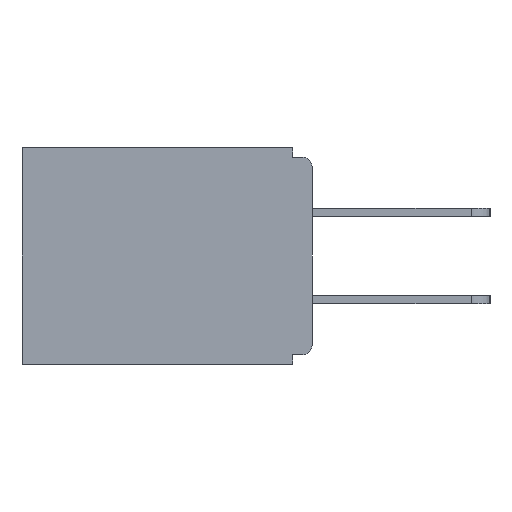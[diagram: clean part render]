
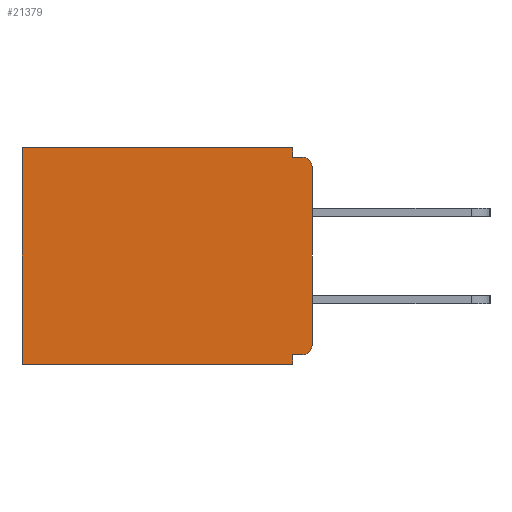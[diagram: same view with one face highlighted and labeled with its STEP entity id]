
A CAD part, left-side view. The second image highlights one B-rep face of the part: STEP entity #21379.
In plain terms, the highlighted planar face has unit normal (-1, 0, 0).
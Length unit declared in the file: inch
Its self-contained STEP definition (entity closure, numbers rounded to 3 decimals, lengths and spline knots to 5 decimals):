
#298 = VERTEX_POINT ( 'NONE', #12669 ) ;
#305 = DIRECTION ( 'NONE',  ( 0., 1., 0. ) ) ;
#724 = EDGE_CURVE ( 'NONE', #17799, #19816, #5233, .T. ) ;
#803 = AXIS2_PLACEMENT_3D ( 'NONE', #21367, #6289, #8257 ) ;
#1035 = DIRECTION ( 'NONE',  ( 0., 0., -1. ) ) ;
#2057 = CARTESIAN_POINT ( 'NONE',  ( 0.298, 0.031, -0.343 ) ) ;
#2880 = VECTOR ( 'NONE', #20160, 39.37008 ) ;
#3311 = DIRECTION ( 'NONE',  ( 0., 0., -1. ) ) ;
#3341 = DIRECTION ( 'NONE',  ( 0., 0., -1. ) ) ;
#4679 = VECTOR ( 'NONE', #11128, 39.37008 ) ;
#5233 = LINE ( 'NONE', #23841, #2880 ) ;
#5255 = CARTESIAN_POINT ( 'NONE',  ( 0.298, 0., 0. ) ) ;
#5290 = DIRECTION ( 'NONE',  ( 0., 0., -1. ) ) ;
#5450 = VECTOR ( 'NONE', #22810, 39.37008 ) ;
#5525 = EDGE_CURVE ( 'NONE', #14277, #6176, #12994, .T. ) ;
#5656 = VECTOR ( 'NONE', #10383, 39.37008 ) ;
#6069 = CARTESIAN_POINT ( 'NONE',  ( 0.298, 0.031, -0.015 ) ) ;
#6142 = LINE ( 'NONE', #14630, #7936 ) ;
#6176 = VERTEX_POINT ( 'NONE', #13397 ) ;
#6250 = EDGE_CURVE ( 'NONE', #19816, #13622, #6320, .T. ) ;
#6289 = DIRECTION ( 'NONE',  ( -1., 0., 0. ) ) ;
#6320 = LINE ( 'NONE', #11673, #5450 ) ;
#6567 = CARTESIAN_POINT ( 'NONE',  ( 0.298, 0.015, -0.328 ) ) ;
#6892 = ORIENTED_EDGE ( 'NONE', *, *, #5525, .T. ) ;
#7248 = CIRCLE ( 'NONE', #803, 0.015 ) ;
#7365 = DIRECTION ( 'NONE',  ( 0., 0., -1. ) ) ;
#7936 = VECTOR ( 'NONE', #5290, 39.37008 ) ;
#8257 = DIRECTION ( 'NONE',  ( 0., 0., -1. ) ) ;
#8286 = AXIS2_PLACEMENT_3D ( 'NONE', #5255, #8669, #3311 ) ;
#8337 = ORIENTED_EDGE ( 'NONE', *, *, #14405, .T. ) ;
#8435 = EDGE_CURVE ( 'NONE', #10183, #6176, #18971, .T. ) ;
#8669 = DIRECTION ( 'NONE',  ( 1., 0., 0. ) ) ;
#9319 = VERTEX_POINT ( 'NONE', #6567 ) ;
#9611 = ORIENTED_EDGE ( 'NONE', *, *, #6250, .F. ) ;
#9703 = CARTESIAN_POINT ( 'NONE',  ( 0.298, 0.46, 0. ) ) ;
#9891 = CARTESIAN_POINT ( 'NONE',  ( 0.298, 0.031, 0. ) ) ;
#10083 = VERTEX_POINT ( 'NONE', #23660 ) ;
#10183 = VERTEX_POINT ( 'NONE', #2057 ) ;
#10383 = DIRECTION ( 'NONE',  ( 0., 1., 0. ) ) ;
#10461 = DIRECTION ( 'NONE',  ( -1., 0., 0. ) ) ;
#11120 = LINE ( 'NONE', #22189, #21811 ) ;
#11128 = DIRECTION ( 'NONE',  ( 0., 1., 0. ) ) ;
#11460 = ORIENTED_EDGE ( 'NONE', *, *, #12858, .T. ) ;
#11673 = CARTESIAN_POINT ( 'NONE',  ( 0.298, 0., -0.015 ) ) ;
#11768 = EDGE_LOOP ( 'NONE', ( #15242, #9611, #22030, #11460, #6892, #17866, #12797, #11913, #8337, #17191 ) ) ;
#11913 = ORIENTED_EDGE ( 'NONE', *, *, #21423, .F. ) ;
#12168 = CARTESIAN_POINT ( 'NONE',  ( 0.298, 0.015, -0.03 ) ) ;
#12349 = CIRCLE ( 'NONE', #21362, 0.015 ) ;
#12669 = CARTESIAN_POINT ( 'NONE',  ( 0.298, 0., -0.03 ) ) ;
#12797 = ORIENTED_EDGE ( 'NONE', *, *, #12963, .F. ) ;
#12858 = EDGE_CURVE ( 'NONE', #17799, #14277, #20676, .T. ) ;
#12963 = EDGE_CURVE ( 'NONE', #14207, #10183, #11120, .T. ) ;
#12994 = LINE ( 'NONE', #18427, #23477 ) ;
#13124 = CARTESIAN_POINT ( 'NONE',  ( 0.298, 0.031, -0.328 ) ) ;
#13397 = CARTESIAN_POINT ( 'NONE',  ( 0.298, 0.46, -0.343 ) ) ;
#13405 = FACE_OUTER_BOUND ( 'NONE', #11768, .T. ) ;
#13622 = VERTEX_POINT ( 'NONE', #22935 ) ;
#14207 = VERTEX_POINT ( 'NONE', #13124 ) ;
#14277 = VERTEX_POINT ( 'NONE', #9703 ) ;
#14405 = EDGE_CURVE ( 'NONE', #9319, #10083, #7248, .T. ) ;
#14630 = CARTESIAN_POINT ( 'NONE',  ( 0.298, 0., 0. ) ) ;
#15242 = ORIENTED_EDGE ( 'NONE', *, *, #15857, .T. ) ;
#15857 = EDGE_CURVE ( 'NONE', #298, #13622, #12349, .T. ) ;
#16037 = PLANE ( 'NONE',  #8286 ) ;
#17191 = ORIENTED_EDGE ( 'NONE', *, *, #20283, .F. ) ;
#17507 = CARTESIAN_POINT ( 'NONE',  ( 0.298, 0., -0.343 ) ) ;
#17799 = VERTEX_POINT ( 'NONE', #9891 ) ;
#17866 = ORIENTED_EDGE ( 'NONE', *, *, #8435, .F. ) ;
#18427 = CARTESIAN_POINT ( 'NONE',  ( 0.298, 0.46, 0. ) ) ;
#18971 = LINE ( 'NONE', #17507, #5656 ) ;
#19816 = VERTEX_POINT ( 'NONE', #6069 ) ;
#20160 = DIRECTION ( 'NONE',  ( 0., 0., -1. ) ) ;
#20283 = EDGE_CURVE ( 'NONE', #298, #10083, #6142, .T. ) ;
#20525 = CARTESIAN_POINT ( 'NONE',  ( 0.298, 0., -0.328 ) ) ;
#20676 = LINE ( 'NONE', #24012, #4679 ) ;
#21362 = AXIS2_PLACEMENT_3D ( 'NONE', #12168, #10461, #1035 ) ;
#21367 = CARTESIAN_POINT ( 'NONE',  ( 0.298, 0.015, -0.313 ) ) ;
#21379 = ADVANCED_FACE ( 'NONE', ( #13405 ), #16037, .F. ) ;
#21423 = EDGE_CURVE ( 'NONE', #9319, #14207, #21483, .T. ) ;
#21483 = LINE ( 'NONE', #20525, #23852 ) ;
#21811 = VECTOR ( 'NONE', #3341, 39.37008 ) ;
#22030 = ORIENTED_EDGE ( 'NONE', *, *, #724, .F. ) ;
#22189 = CARTESIAN_POINT ( 'NONE',  ( 0.298, 0.031, -0.343 ) ) ;
#22810 = DIRECTION ( 'NONE',  ( 0., -1., 0. ) ) ;
#22935 = CARTESIAN_POINT ( 'NONE',  ( 0.298, 0.015, -0.015 ) ) ;
#23477 = VECTOR ( 'NONE', #7365, 39.37008 ) ;
#23660 = CARTESIAN_POINT ( 'NONE',  ( 0.298, 0., -0.313 ) ) ;
#23841 = CARTESIAN_POINT ( 'NONE',  ( 0.298, 0.031, -0.343 ) ) ;
#23852 = VECTOR ( 'NONE', #305, 39.37008 ) ;
#24012 = CARTESIAN_POINT ( 'NONE',  ( 0.298, 0., 0. ) ) ;
